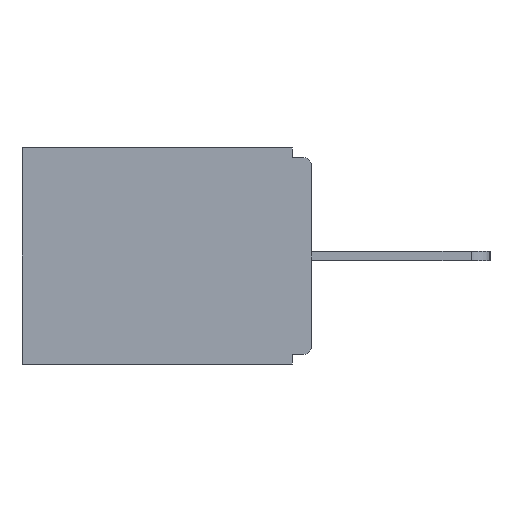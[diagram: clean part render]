
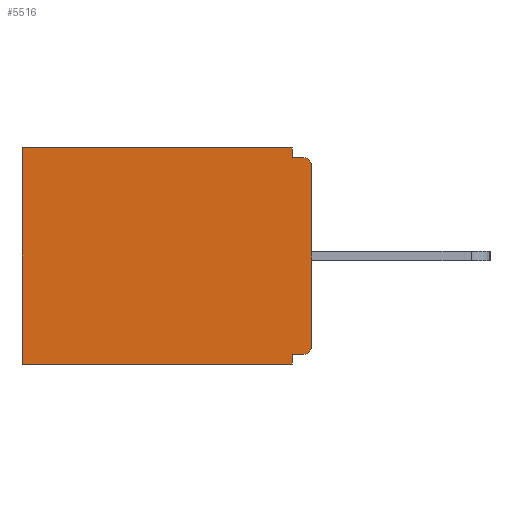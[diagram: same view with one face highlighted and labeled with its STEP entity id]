
A CAD part, left-side view. The second image highlights one B-rep face of the part: STEP entity #5516.
In plain terms, the highlighted planar face has unit normal (-1, 0, 0).
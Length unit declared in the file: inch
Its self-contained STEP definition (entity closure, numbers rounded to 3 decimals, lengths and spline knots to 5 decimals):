
#83 = EDGE_CURVE ( 'NONE', #12406, #13797, #12335, .T. ) ;
#168 = VECTOR ( 'NONE', #8545, 39.37008 ) ;
#202 = CARTESIAN_POINT ( 'NONE',  ( 0.298, 0.031, -0.343 ) ) ;
#238 = VECTOR ( 'NONE', #795, 39.37008 ) ;
#408 = DIRECTION ( 'NONE',  ( 0., 0., -1. ) ) ;
#429 = ORIENTED_EDGE ( 'NONE', *, *, #5498, .F. ) ;
#509 = ORIENTED_EDGE ( 'NONE', *, *, #10642, .F. ) ;
#600 = EDGE_CURVE ( 'NONE', #14246, #5924, #8055, .T. ) ;
#795 = DIRECTION ( 'NONE',  ( 0., -1., 0. ) ) ;
#870 = EDGE_CURVE ( 'NONE', #6563, #13809, #13350, .T. ) ;
#1071 = CARTESIAN_POINT ( 'NONE',  ( 0.298, 0.031, 0. ) ) ;
#1431 = DIRECTION ( 'NONE',  ( 0., 0., -1. ) ) ;
#1523 = DIRECTION ( 'NONE',  ( 0., 0., -1. ) ) ;
#1977 = CIRCLE ( 'NONE', #3656, 0.015 ) ;
#1978 = CARTESIAN_POINT ( 'NONE',  ( 0.298, 0.46, 0. ) ) ;
#2282 = ORIENTED_EDGE ( 'NONE', *, *, #10454, .T. ) ;
#2461 = CARTESIAN_POINT ( 'NONE',  ( 0.298, 0.46, -0.343 ) ) ;
#2496 = VERTEX_POINT ( 'NONE', #12656 ) ;
#2605 = VECTOR ( 'NONE', #408, 39.37008 ) ;
#2712 = DIRECTION ( 'NONE',  ( 0., 1., 0. ) ) ;
#2894 = CARTESIAN_POINT ( 'NONE',  ( 0.298, 0., 0. ) ) ;
#2903 = VERTEX_POINT ( 'NONE', #8299 ) ;
#3656 = AXIS2_PLACEMENT_3D ( 'NONE', #11786, #14061, #1431 ) ;
#3768 = CARTESIAN_POINT ( 'NONE',  ( 0.298, 0.031, -0.343 ) ) ;
#4022 = DIRECTION ( 'NONE',  ( 0., 1., 0. ) ) ;
#4067 = VERTEX_POINT ( 'NONE', #6423 ) ;
#4143 = LINE ( 'NONE', #10872, #168 ) ;
#4168 = CARTESIAN_POINT ( 'NONE',  ( 0.298, 0., -0.015 ) ) ;
#4569 = DIRECTION ( 'NONE',  ( 0., 0., -1. ) ) ;
#4611 = LINE ( 'NONE', #3768, #8170 ) ;
#4947 = VECTOR ( 'NONE', #2712, 39.37008 ) ;
#4966 = ORIENTED_EDGE ( 'NONE', *, *, #8931, .T. ) ;
#5093 = VECTOR ( 'NONE', #5357, 39.37008 ) ;
#5153 = EDGE_CURVE ( 'NONE', #2496, #4067, #13048, .T. ) ;
#5357 = DIRECTION ( 'NONE',  ( 0., 0., -1. ) ) ;
#5398 = CARTESIAN_POINT ( 'NONE',  ( 0.298, 0., -0.343 ) ) ;
#5498 = EDGE_CURVE ( 'NONE', #11942, #6563, #4611, .T. ) ;
#5516 = ADVANCED_FACE ( 'NONE', ( #14151 ), #11654, .F. ) ;
#5589 = CARTESIAN_POINT ( 'NONE',  ( 0.298, 0.031, -0.343 ) ) ;
#5924 = VERTEX_POINT ( 'NONE', #5589 ) ;
#6326 = VECTOR ( 'NONE', #4022, 39.37008 ) ;
#6360 = EDGE_LOOP ( 'NONE', ( #11370, #10931, #429, #4966, #12425, #509, #8980, #11193, #2282, #14069 ) ) ;
#6423 = CARTESIAN_POINT ( 'NONE',  ( 0.298, 0., -0.313 ) ) ;
#6445 = LINE ( 'NONE', #2894, #6326 ) ;
#6563 = VERTEX_POINT ( 'NONE', #14706 ) ;
#7341 = CARTESIAN_POINT ( 'NONE',  ( 0.298, 0., 0. ) ) ;
#8055 = LINE ( 'NONE', #202, #13249 ) ;
#8170 = VECTOR ( 'NONE', #1523, 39.37008 ) ;
#8249 = DIRECTION ( 'NONE',  ( 0., 0., -1. ) ) ;
#8299 = CARTESIAN_POINT ( 'NONE',  ( 0.298, 0.015, -0.328 ) ) ;
#8483 = EDGE_CURVE ( 'NONE', #2496, #13809, #1977, .T. ) ;
#8545 = DIRECTION ( 'NONE',  ( 0., 1., 0. ) ) ;
#8931 = EDGE_CURVE ( 'NONE', #11942, #12406, #6445, .T. ) ;
#8980 = ORIENTED_EDGE ( 'NONE', *, *, #600, .F. ) ;
#9160 = DIRECTION ( 'NONE',  ( -1., 0., 0. ) ) ;
#9179 = CARTESIAN_POINT ( 'NONE',  ( 0.298, 0.031, -0.328 ) ) ;
#10454 = EDGE_CURVE ( 'NONE', #2903, #4067, #14391, .T. ) ;
#10567 = AXIS2_PLACEMENT_3D ( 'NONE', #7341, #11949, #8249 ) ;
#10569 = DIRECTION ( 'NONE',  ( 0., 0., -1. ) ) ;
#10588 = CARTESIAN_POINT ( 'NONE',  ( 0.298, 0., 0. ) ) ;
#10642 = EDGE_CURVE ( 'NONE', #5924, #13797, #12306, .T. ) ;
#10872 = CARTESIAN_POINT ( 'NONE',  ( 0.298, 0., -0.328 ) ) ;
#10931 = ORIENTED_EDGE ( 'NONE', *, *, #870, .F. ) ;
#10975 = AXIS2_PLACEMENT_3D ( 'NONE', #12799, #9160, #10569 ) ;
#11193 = ORIENTED_EDGE ( 'NONE', *, *, #11722, .F. ) ;
#11370 = ORIENTED_EDGE ( 'NONE', *, *, #8483, .T. ) ;
#11543 = CARTESIAN_POINT ( 'NONE',  ( 0.298, 0.015, -0.015 ) ) ;
#11654 = PLANE ( 'NONE',  #10567 ) ;
#11722 = EDGE_CURVE ( 'NONE', #2903, #14246, #4143, .T. ) ;
#11786 = CARTESIAN_POINT ( 'NONE',  ( 0.298, 0.015, -0.03 ) ) ;
#11942 = VERTEX_POINT ( 'NONE', #1071 ) ;
#11949 = DIRECTION ( 'NONE',  ( 1., 0., 0. ) ) ;
#12306 = LINE ( 'NONE', #5398, #4947 ) ;
#12335 = LINE ( 'NONE', #1978, #5093 ) ;
#12406 = VERTEX_POINT ( 'NONE', #13532 ) ;
#12425 = ORIENTED_EDGE ( 'NONE', *, *, #83, .T. ) ;
#12656 = CARTESIAN_POINT ( 'NONE',  ( 0.298, 0., -0.03 ) ) ;
#12799 = CARTESIAN_POINT ( 'NONE',  ( 0.298, 0.015, -0.313 ) ) ;
#13048 = LINE ( 'NONE', #10588, #2605 ) ;
#13249 = VECTOR ( 'NONE', #4569, 39.37008 ) ;
#13350 = LINE ( 'NONE', #4168, #238 ) ;
#13532 = CARTESIAN_POINT ( 'NONE',  ( 0.298, 0.46, 0. ) ) ;
#13797 = VERTEX_POINT ( 'NONE', #2461 ) ;
#13809 = VERTEX_POINT ( 'NONE', #11543 ) ;
#14061 = DIRECTION ( 'NONE',  ( -1., 0., 0. ) ) ;
#14069 = ORIENTED_EDGE ( 'NONE', *, *, #5153, .F. ) ;
#14151 = FACE_OUTER_BOUND ( 'NONE', #6360, .T. ) ;
#14246 = VERTEX_POINT ( 'NONE', #9179 ) ;
#14391 = CIRCLE ( 'NONE', #10975, 0.015 ) ;
#14706 = CARTESIAN_POINT ( 'NONE',  ( 0.298, 0.031, -0.015 ) ) ;
